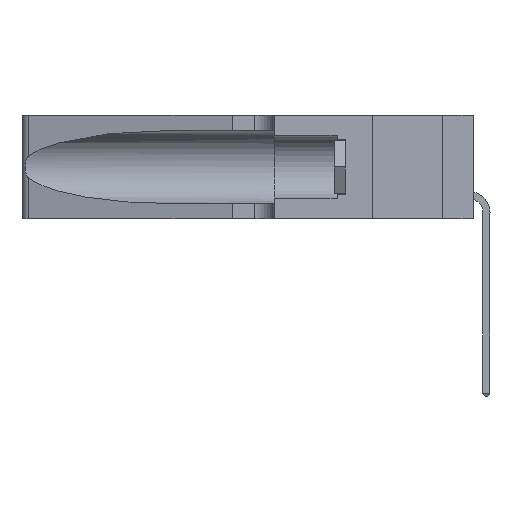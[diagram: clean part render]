
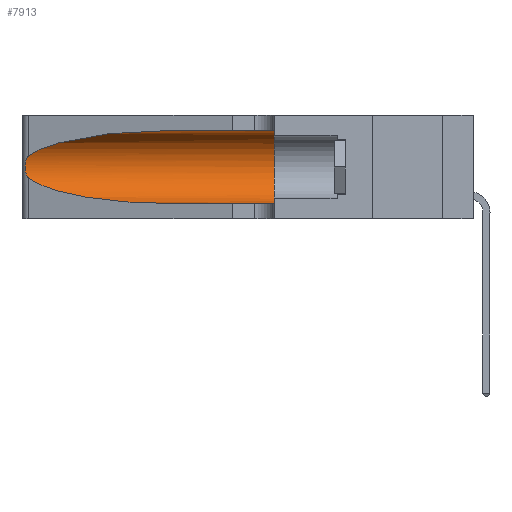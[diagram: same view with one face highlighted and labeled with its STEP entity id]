
A CAD part, left-side view. The second image highlights one B-rep face of the part: STEP entity #7913.
In plain terms, the highlighted cylindrical face has radius 3.308 mm (diameter 6.617 mm), a partial arc.
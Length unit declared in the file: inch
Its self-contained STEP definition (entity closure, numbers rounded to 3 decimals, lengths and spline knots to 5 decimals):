
#269 = CARTESIAN_POINT ( 'NONE',  ( 0.25555, 1.22994, 0.2215 ) ) ;
#395 = CARTESIAN_POINT ( 'NONE',  ( 0.1305, 1.61858, 0.05475 ) ) ;
#1539 = CARTESIAN_POINT ( 'NONE',  ( 0.1305, 0.35, 0.31525 ) ) ;
#1563 = B_SPLINE_CURVE_WITH_KNOTS ( 'NONE', 3,
 ( #20957, #269, #14896, #16736, #22922, #14540, #20863, #27149, #12539, #21053, #2022, #23118, #14718, #2199 ),
 .UNSPECIFIED., .F., .F.,
 ( 4, 2, 2, 2, 2, 2, 4 ),
 ( 0., 0.00027, 0.00053, 0.00107, 0.0016, 0.00187, 0.00214 ),
 .UNSPECIFIED. ) ;
#1953 = ORIENTED_EDGE ( 'NONE', *, *, #16796, .T. ) ;
#2022 = CARTESIAN_POINT ( 'NONE',  ( 0.25789, 1.23486, 0.15765 ) ) ;
#2096 = CARTESIAN_POINT ( 'NONE',  ( 0.1305, 0.35, 0.05475 ) ) ;
#2199 = CARTESIAN_POINT ( 'NONE',  ( 0.25487, 1.22718, 0.14631 ) ) ;
#2602 = VERTEX_POINT ( 'NONE', #1539 ) ;
#2735 = CARTESIAN_POINT ( 'NONE',  ( 0.1305, 0.35, 0.185 ) ) ;
#3277 = CARTESIAN_POINT ( 'NONE',  ( 0.2373, 1.15595, 0.08982 ) ) ;
#4081 =( BOUNDED_CURVE ( )  B_SPLINE_CURVE ( 3, ( #8757, #12678, #10754, #25448 ),
 .UNSPECIFIED., .F., .F. ) 
 B_SPLINE_CURVE_WITH_KNOTS ( ( 4, 4 ),
 ( 1.5708, 2.84003 ),
 .UNSPECIFIED. ) 
 CURVE ( )  GEOMETRIC_REPRESENTATION_ITEM ( )  RATIONAL_B_SPLINE_CURVE ( ( 1., 0.87, 0.87, 1. ) ) 
 REPRESENTATION_ITEM ( '' )  );
#4585 = VERTEX_POINT ( 'NONE', #12098 ) ;
#4644 = CARTESIAN_POINT ( 'NONE',  ( 0.1305, 0.72297, 0.05475 ) ) ;
#4862 = AXIS2_PLACEMENT_3D ( 'NONE', #2735, #21410, #21224 ) ;
#5271 =( BOUNDED_CURVE ( )  B_SPLINE_CURVE ( 3, ( #13314, #3277, #7113, #7401 ),
 .UNSPECIFIED., .F., .F. ) 
 B_SPLINE_CURVE_WITH_KNOTS ( ( 4, 4 ),
 ( 3.44316, 4.71239 ),
 .UNSPECIFIED. ) 
 CURVE ( )  GEOMETRIC_REPRESENTATION_ITEM ( )  RATIONAL_B_SPLINE_CURVE ( ( 1., 0.87, 0.87, 1. ) ) 
 REPRESENTATION_ITEM ( '' )  );
#5660 = FACE_OUTER_BOUND ( 'NONE', #21644, .T. ) ;
#6831 = VERTEX_POINT ( 'NONE', #2096 ) ;
#6957 = CIRCLE ( 'NONE', #4862, 0.13025 ) ;
#7113 = CARTESIAN_POINT ( 'NONE',  ( 0.18966, 0.96281, 0.05475 ) ) ;
#7401 = CARTESIAN_POINT ( 'NONE',  ( 0.1305, 0.72297, 0.05475 ) ) ;
#7907 = CARTESIAN_POINT ( 'NONE',  ( 0.1305, 1.61858, 0.185 ) ) ;
#7913 = ADVANCED_FACE ( 'NONE', ( #5660 ), #23033, .F. ) ;
#8543 = ORIENTED_EDGE ( 'NONE', *, *, #17679, .T. ) ;
#8757 = CARTESIAN_POINT ( 'NONE',  ( 0.1305, 0.72297, 0.31525 ) ) ;
#9087 = CARTESIAN_POINT ( 'NONE',  ( 0.25487, 1.22718, 0.22369 ) ) ;
#9636 = VERTEX_POINT ( 'NONE', #9087 ) ;
#10637 = LINE ( 'NONE', #26519, #12607 ) ;
#10754 = CARTESIAN_POINT ( 'NONE',  ( 0.2373, 1.15595, 0.28018 ) ) ;
#11161 = ORIENTED_EDGE ( 'NONE', *, *, #11953, .T. ) ;
#11349 = EDGE_CURVE ( 'NONE', #9636, #24248, #1563, .T. ) ;
#11472 = EDGE_CURVE ( 'NONE', #2602, #6831, #6957, .T. ) ;
#11953 = EDGE_CURVE ( 'NONE', #4585, #9636, #4081, .T. ) ;
#12098 = CARTESIAN_POINT ( 'NONE',  ( 0.1305, 0.72297, 0.31525 ) ) ;
#12539 = CARTESIAN_POINT ( 'NONE',  ( 0.26017, 1.23833, 0.17102 ) ) ;
#12607 = VECTOR ( 'NONE', #18407, 39.37008 ) ;
#12678 = CARTESIAN_POINT ( 'NONE',  ( 0.18966, 0.96281, 0.31525 ) ) ;
#13314 = CARTESIAN_POINT ( 'NONE',  ( 0.25487, 1.22718, 0.14631 ) ) ;
#14206 = DIRECTION ( 'NONE',  ( 0., 0., -1. ) ) ;
#14540 = CARTESIAN_POINT ( 'NONE',  ( 0.26018, 1.23835, 0.19895 ) ) ;
#14718 = CARTESIAN_POINT ( 'NONE',  ( 0.25555, 1.22993, 0.14849 ) ) ;
#14896 = CARTESIAN_POINT ( 'NONE',  ( 0.25639, 1.23184, 0.21858 ) ) ;
#14977 = EDGE_CURVE ( 'NONE', #4585, #2602, #10637, .T. ) ;
#15007 = DIRECTION ( 'NONE',  ( 0., -1., 0. ) ) ;
#15766 = ORIENTED_EDGE ( 'NONE', *, *, #11349, .T. ) ;
#16736 = CARTESIAN_POINT ( 'NONE',  ( 0.25787, 1.23484, 0.2124 ) ) ;
#16796 = EDGE_CURVE ( 'NONE', #24248, #22461, #5271, .T. ) ;
#17011 = ORIENTED_EDGE ( 'NONE', *, *, #11472, .F. ) ;
#17679 = EDGE_CURVE ( 'NONE', #22461, #6831, #21942, .T. ) ;
#18407 = DIRECTION ( 'NONE',  ( 0., -1., 0. ) ) ;
#18831 = CARTESIAN_POINT ( 'NONE',  ( 0.25487, 1.22718, 0.14631 ) ) ;
#20863 = CARTESIAN_POINT ( 'NONE',  ( 0.26075, 1.23896, 0.19203 ) ) ;
#20957 = CARTESIAN_POINT ( 'NONE',  ( 0.25487, 1.22718, 0.22369 ) ) ;
#21053 = CARTESIAN_POINT ( 'NONE',  ( 0.25856, 1.23593, 0.16098 ) ) ;
#21224 = DIRECTION ( 'NONE',  ( 0., 0., 1. ) ) ;
#21410 = DIRECTION ( 'NONE',  ( 0., 1., 0. ) ) ;
#21644 = EDGE_LOOP ( 'NONE', ( #11161, #15766, #1953, #8543, #17011, #25393 ) ) ;
#21942 = LINE ( 'NONE', #395, #22297 ) ;
#22297 = VECTOR ( 'NONE', #15007, 39.37008 ) ;
#22461 = VERTEX_POINT ( 'NONE', #4644 ) ;
#22922 = CARTESIAN_POINT ( 'NONE',  ( 0.25854, 1.2359, 0.20912 ) ) ;
#23033 = CYLINDRICAL_SURFACE ( 'NONE', #24139, 0.13025 ) ;
#23118 = CARTESIAN_POINT ( 'NONE',  ( 0.25639, 1.23186, 0.15144 ) ) ;
#24139 = AXIS2_PLACEMENT_3D ( 'NONE', #7907, #26710, #14206 ) ;
#24248 = VERTEX_POINT ( 'NONE', #18831 ) ;
#25393 = ORIENTED_EDGE ( 'NONE', *, *, #14977, .F. ) ;
#25448 = CARTESIAN_POINT ( 'NONE',  ( 0.25487, 1.22718, 0.22369 ) ) ;
#26519 = CARTESIAN_POINT ( 'NONE',  ( 0.1305, 1.61858, 0.31525 ) ) ;
#26710 = DIRECTION ( 'NONE',  ( 0., -1., 0. ) ) ;
#27149 = CARTESIAN_POINT ( 'NONE',  ( 0.26075, 1.23896, 0.178 ) ) ;
